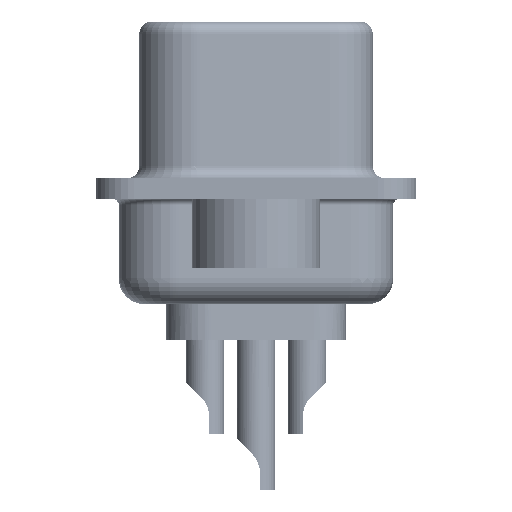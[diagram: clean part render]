
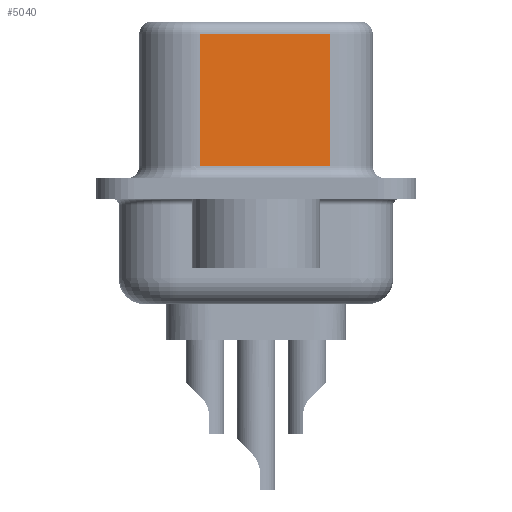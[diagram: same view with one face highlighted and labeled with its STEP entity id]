
A CAD part, left-side view. The second image highlights one B-rep face of the part: STEP entity #5040.
In plain terms, the highlighted planar face has unit normal (-0.985, -0.174, 0).
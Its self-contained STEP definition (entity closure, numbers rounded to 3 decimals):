
#498 = CARTESIAN_POINT ( 'NONE',  ( 4.58, -2.897, 6.02 ) ) ;
#2179 = ORIENTED_EDGE ( 'NONE', *, *, #9988, .F. ) ;
#2434 = DIRECTION ( 'NONE',  ( 0.174, -0.985, 0. ) ) ;
#3282 = VECTOR ( 'NONE', #12229, 1000. ) ;
#4573 = DIRECTION ( 'NONE',  ( -0.174, 0.985, 0. ) ) ;
#4685 = ORIENTED_EDGE ( 'NONE', *, *, #7803, .T. ) ;
#5040 = ADVANCED_FACE ( 'NONE', ( #20165 ), #24342, .F. ) ;
#5707 = LINE ( 'NONE', #27061, #23606 ) ;
#5741 = ORIENTED_EDGE ( 'NONE', *, *, #32680, .T. ) ;
#6600 = VERTEX_POINT ( 'NONE', #498 ) ;
#7630 = EDGE_LOOP ( 'NONE', ( #2179, #5741, #10797, #4685 ) ) ;
#7803 = EDGE_CURVE ( 'NONE', #9143, #24028, #16294, .T. ) ;
#7927 = CARTESIAN_POINT ( 'NONE',  ( 3.68, 2.203, 0.9 ) ) ;
#9143 = VERTEX_POINT ( 'NONE', #7927 ) ;
#9634 = CARTESIAN_POINT ( 'NONE',  ( 3.68, 2.203, 6.52 ) ) ;
#9988 = EDGE_CURVE ( 'NONE', #6600, #24028, #30164, .T. ) ;
#10034 = AXIS2_PLACEMENT_3D ( 'NONE', #20890, #24276, #4573 ) ;
#10797 = ORIENTED_EDGE ( 'NONE', *, *, #28064, .T. ) ;
#10996 = LINE ( 'NONE', #9634, #3282 ) ;
#12058 = DIRECTION ( 'NONE',  ( -0.174, 0.985, 0. ) ) ;
#12229 = DIRECTION ( 'NONE',  ( 0., 0., -1. ) ) ;
#14774 = DIRECTION ( 'NONE',  ( 0., 0., -1. ) ) ;
#15501 = VECTOR ( 'NONE', #2434, 1000. ) ;
#16246 = VERTEX_POINT ( 'NONE', #32094 ) ;
#16294 = LINE ( 'NONE', #32668, #15501 ) ;
#17266 = CARTESIAN_POINT ( 'NONE',  ( 4.58, -2.897, 6.52 ) ) ;
#20165 = FACE_OUTER_BOUND ( 'NONE', #7630, .T. ) ;
#20890 = CARTESIAN_POINT ( 'NONE',  ( 4.58, -2.897, 6.52 ) ) ;
#22031 = VECTOR ( 'NONE', #14774, 1000. ) ;
#23606 = VECTOR ( 'NONE', #12058, 1000. ) ;
#24028 = VERTEX_POINT ( 'NONE', #29585 ) ;
#24276 = DIRECTION ( 'NONE',  ( 0.985, 0.174, 0. ) ) ;
#24342 = PLANE ( 'NONE',  #10034 ) ;
#27061 = CARTESIAN_POINT ( 'NONE',  ( 4.58, -2.897, 6.02 ) ) ;
#28064 = EDGE_CURVE ( 'NONE', #16246, #9143, #10996, .T. ) ;
#29585 = CARTESIAN_POINT ( 'NONE',  ( 4.58, -2.897, 0.9 ) ) ;
#30164 = LINE ( 'NONE', #17266, #22031 ) ;
#32094 = CARTESIAN_POINT ( 'NONE',  ( 3.68, 2.203, 6.02 ) ) ;
#32668 = CARTESIAN_POINT ( 'NONE',  ( 4.58, -2.897, 0.9 ) ) ;
#32680 = EDGE_CURVE ( 'NONE', #6600, #16246, #5707, .T. ) ;
